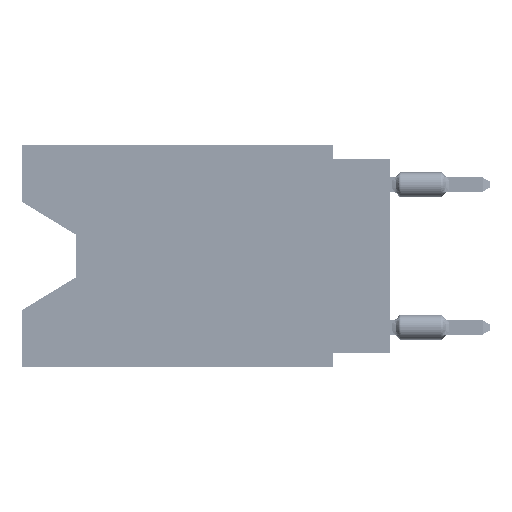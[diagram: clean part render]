
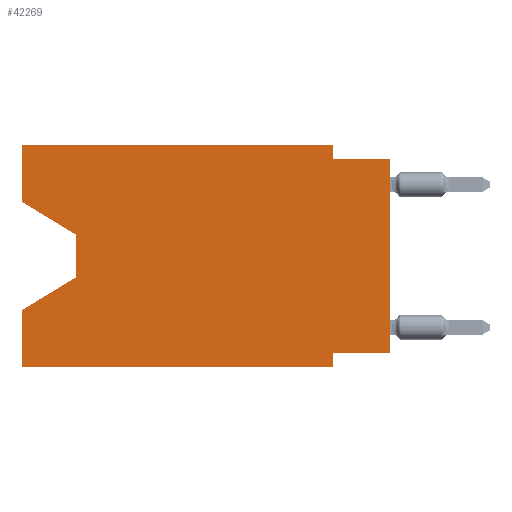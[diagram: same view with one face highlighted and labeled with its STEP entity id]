
A CAD part, left-side view. The second image highlights one B-rep face of the part: STEP entity #42269.
In plain terms, the highlighted planar face has unit normal (-1, 0, 0).
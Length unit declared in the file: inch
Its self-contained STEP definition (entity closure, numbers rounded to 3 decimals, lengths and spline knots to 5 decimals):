
#289 = CARTESIAN_POINT ( 'NONE',  ( 0., 0.1, 0. ) ) ;
#880 = VERTEX_POINT ( 'NONE', #4536 ) ;
#1342 = ORIENTED_EDGE ( 'NONE', *, *, #11553, .F. ) ;
#1544 = EDGE_CURVE ( 'NONE', #46115, #29240, #26456, .T. ) ;
#1562 = LINE ( 'NONE', #10378, #17788 ) ;
#1723 = ORIENTED_EDGE ( 'NONE', *, *, #2730, .F. ) ;
#2730 = EDGE_CURVE ( 'NONE', #24843, #28762, #7207, .T. ) ;
#4258 = EDGE_LOOP ( 'NONE', ( #5756, #21449, #30472, #33314, #34497, #44040, #1723, #50771, #1342, #31789, #10161, #5428 ) ) ;
#4536 = CARTESIAN_POINT ( 'NONE',  ( 0., 0.645, -0.10025 ) ) ;
#4874 = VERTEX_POINT ( 'NONE', #38742 ) ;
#5428 = ORIENTED_EDGE ( 'NONE', *, *, #38190, .F. ) ;
#5484 = CARTESIAN_POINT ( 'NONE',  ( 0., 0., -0.365 ) ) ;
#5756 = ORIENTED_EDGE ( 'NONE', *, *, #16462, .T. ) ;
#6175 = DIRECTION ( 'NONE',  ( 0., 0., 1. ) ) ;
#7207 = LINE ( 'NONE', #21843, #35158 ) ;
#7209 = DIRECTION ( 'NONE',  ( 0., 0., -1. ) ) ;
#7213 = VECTOR ( 'NONE', #53474, 39.37008 ) ;
#7805 = DIRECTION ( 'NONE',  ( 0., 0., 1. ) ) ;
#10161 = ORIENTED_EDGE ( 'NONE', *, *, #26925, .F. ) ;
#10378 = CARTESIAN_POINT ( 'NONE',  ( 0., 0.55, -0.232 ) ) ;
#10557 = LINE ( 'NONE', #46652, #50993 ) ;
#10811 = DIRECTION ( 'NONE',  ( 1., 0., 0. ) ) ;
#11553 = EDGE_CURVE ( 'NONE', #49460, #23619, #10557, .T. ) ;
#11814 = CARTESIAN_POINT ( 'NONE',  ( 0., 0.55, -0.232 ) ) ;
#11888 = LINE ( 'NONE', #28907, #47583 ) ;
#12380 = CARTESIAN_POINT ( 'NONE',  ( 0., 0.645, -0.39 ) ) ;
#12624 = LINE ( 'NONE', #289, #30596 ) ;
#13495 = DIRECTION ( 'NONE',  ( 0., 0., 1. ) ) ;
#14164 = LINE ( 'NONE', #55747, #50602 ) ;
#14616 = EDGE_CURVE ( 'NONE', #28751, #49460, #12624, .T. ) ;
#15606 = VECTOR ( 'NONE', #7805, 39.37008 ) ;
#16374 = CARTESIAN_POINT ( 'NONE',  ( 0., 0., -0.025 ) ) ;
#16462 = EDGE_CURVE ( 'NONE', #880, #41196, #23672, .T. ) ;
#17596 = CARTESIAN_POINT ( 'NONE',  ( 0., 0.1, -0.365 ) ) ;
#17788 = VECTOR ( 'NONE', #36783, 39.37008 ) ;
#17878 = CARTESIAN_POINT ( 'NONE',  ( 0., 0.1, 0. ) ) ;
#18188 = CARTESIAN_POINT ( 'NONE',  ( 0., 0.645, 0. ) ) ;
#19917 = VERTEX_POINT ( 'NONE', #11814 ) ;
#20199 = FACE_OUTER_BOUND ( 'NONE', #4258, .T. ) ;
#21449 = ORIENTED_EDGE ( 'NONE', *, *, #48249, .T. ) ;
#21843 = CARTESIAN_POINT ( 'NONE',  ( 0., 0., -0.365 ) ) ;
#22587 = DIRECTION ( 'NONE',  ( 0., 0., -1. ) ) ;
#22751 = EDGE_CURVE ( 'NONE', #28762, #29240, #11888, .T. ) ;
#23619 = VERTEX_POINT ( 'NONE', #16374 ) ;
#23672 = LINE ( 'NONE', #50681, #50445 ) ;
#24843 = VERTEX_POINT ( 'NONE', #5484 ) ;
#26456 = LINE ( 'NONE', #12380, #7213 ) ;
#26925 = EDGE_CURVE ( 'NONE', #29296, #28751, #14164, .T. ) ;
#28311 = CARTESIAN_POINT ( 'NONE',  ( 0., 0.55, -0.158 ) ) ;
#28751 = VERTEX_POINT ( 'NONE', #17878 ) ;
#28762 = VERTEX_POINT ( 'NONE', #17596 ) ;
#28907 = CARTESIAN_POINT ( 'NONE',  ( 0., 0.1, -0.39 ) ) ;
#29240 = VERTEX_POINT ( 'NONE', #40382 ) ;
#29276 = DIRECTION ( 'NONE',  ( 0., 0., -1. ) ) ;
#29296 = VERTEX_POINT ( 'NONE', #37703 ) ;
#30423 = CARTESIAN_POINT ( 'NONE',  ( 0., 0.55, -0.158 ) ) ;
#30472 = ORIENTED_EDGE ( 'NONE', *, *, #47596, .T. ) ;
#30596 = VECTOR ( 'NONE', #22587, 39.37008 ) ;
#30953 = VECTOR ( 'NONE', #42979, 39.37008 ) ;
#31789 = ORIENTED_EDGE ( 'NONE', *, *, #14616, .F. ) ;
#32868 = LINE ( 'NONE', #50791, #37056 ) ;
#33314 = ORIENTED_EDGE ( 'NONE', *, *, #33506, .F. ) ;
#33506 = EDGE_CURVE ( 'NONE', #46115, #4874, #41344, .T. ) ;
#34468 = DIRECTION ( 'NONE',  ( 0., 1., 0. ) ) ;
#34497 = ORIENTED_EDGE ( 'NONE', *, *, #1544, .T. ) ;
#34773 = LINE ( 'NONE', #38599, #15606 ) ;
#35158 = VECTOR ( 'NONE', #34468, 39.37008 ) ;
#36783 = DIRECTION ( 'NONE',  ( 0., 0.855, -0.519 ) ) ;
#37056 = VECTOR ( 'NONE', #6175, 39.37008 ) ;
#37703 = CARTESIAN_POINT ( 'NONE',  ( 0., 0.645, 0. ) ) ;
#38090 = PLANE ( 'NONE',  #48447 ) ;
#38190 = EDGE_CURVE ( 'NONE', #880, #29296, #34773, .T. ) ;
#38599 = CARTESIAN_POINT ( 'NONE',  ( 0., 0.645, 0. ) ) ;
#38742 = CARTESIAN_POINT ( 'NONE',  ( 0., 0.645, -0.28975 ) ) ;
#40382 = CARTESIAN_POINT ( 'NONE',  ( 0., 0.1, -0.39 ) ) ;
#40647 = EDGE_CURVE ( 'NONE', #24843, #23619, #32868, .T. ) ;
#41196 = VERTEX_POINT ( 'NONE', #30423 ) ;
#41344 = LINE ( 'NONE', #18188, #51754 ) ;
#42269 = ADVANCED_FACE ( 'NONE', ( #20199 ), #38090, .F. ) ;
#42979 = DIRECTION ( 'NONE',  ( 0., 0., -1. ) ) ;
#44040 = ORIENTED_EDGE ( 'NONE', *, *, #22751, .F. ) ;
#46070 = DIRECTION ( 'NONE',  ( 0., -1., 0. ) ) ;
#46115 = VERTEX_POINT ( 'NONE', #53482 ) ;
#46642 = DIRECTION ( 'NONE',  ( 0., -1., 0. ) ) ;
#46652 = CARTESIAN_POINT ( 'NONE',  ( 0., 0., -0.025 ) ) ;
#47583 = VECTOR ( 'NONE', #7209, 39.37008 ) ;
#47596 = EDGE_CURVE ( 'NONE', #19917, #4874, #1562, .T. ) ;
#48249 = EDGE_CURVE ( 'NONE', #41196, #19917, #51512, .T. ) ;
#48447 = AXIS2_PLACEMENT_3D ( 'NONE', #51614, #10811, #29276 ) ;
#49120 = CARTESIAN_POINT ( 'NONE',  ( 0., 0.1, -0.025 ) ) ;
#49460 = VERTEX_POINT ( 'NONE', #49120 ) ;
#50108 = DIRECTION ( 'NONE',  ( 0., -0.855, -0.519 ) ) ;
#50445 = VECTOR ( 'NONE', #50108, 39.37008 ) ;
#50602 = VECTOR ( 'NONE', #46642, 39.37008 ) ;
#50681 = CARTESIAN_POINT ( 'NONE',  ( 0., 0.645, -0.10025 ) ) ;
#50771 = ORIENTED_EDGE ( 'NONE', *, *, #40647, .T. ) ;
#50791 = CARTESIAN_POINT ( 'NONE',  ( 0., 0., 0. ) ) ;
#50993 = VECTOR ( 'NONE', #46070, 39.37008 ) ;
#51512 = LINE ( 'NONE', #28311, #30953 ) ;
#51614 = CARTESIAN_POINT ( 'NONE',  ( 0., 0.645, 0. ) ) ;
#51754 = VECTOR ( 'NONE', #13495, 39.37008 ) ;
#53474 = DIRECTION ( 'NONE',  ( 0., -1., 0. ) ) ;
#53482 = CARTESIAN_POINT ( 'NONE',  ( 0., 0.645, -0.39 ) ) ;
#55747 = CARTESIAN_POINT ( 'NONE',  ( 0., 0.645, 0. ) ) ;
